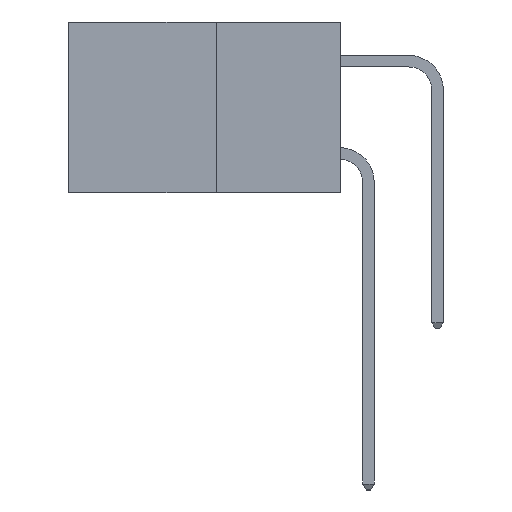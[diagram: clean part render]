
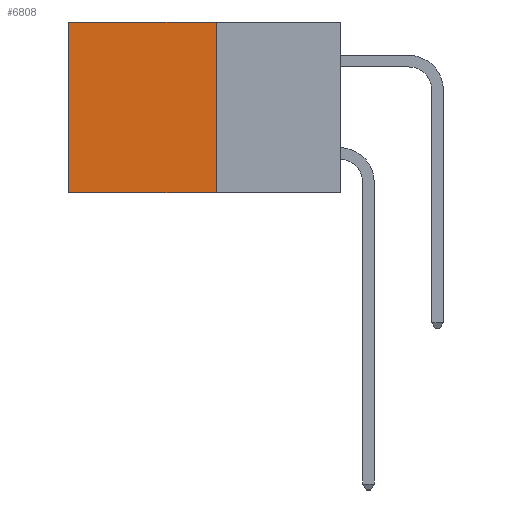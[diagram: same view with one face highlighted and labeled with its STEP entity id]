
A CAD part, left-side view. The second image highlights one B-rep face of the part: STEP entity #6808.
In plain terms, the highlighted planar face has unit normal (-1, 0, 0).
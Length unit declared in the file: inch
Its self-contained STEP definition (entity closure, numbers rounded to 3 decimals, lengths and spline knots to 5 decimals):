
#456 = EDGE_CURVE ( 'NONE', #7021, #8638, #703, .T. ) ;
#476 = VECTOR ( 'NONE', #827, 39.37008 ) ;
#616 = CARTESIAN_POINT ( 'NONE',  ( 0.277, 0.27, -0.37 ) ) ;
#703 = LINE ( 'NONE', #6790, #476 ) ;
#827 = DIRECTION ( 'NONE',  ( 0., 0., -1. ) ) ;
#1119 = VECTOR ( 'NONE', #8045, 39.37008 ) ;
#1345 = LINE ( 'NONE', #4326, #1119 ) ;
#1352 = DIRECTION ( 'NONE',  ( 0., 0., -1. ) ) ;
#1449 = LINE ( 'NONE', #4760, #7214 ) ;
#1884 = VERTEX_POINT ( 'NONE', #9195 ) ;
#2374 = DIRECTION ( 'NONE',  ( 0., 0., -1. ) ) ;
#2786 = AXIS2_PLACEMENT_3D ( 'NONE', #616, #5865, #1352 ) ;
#3178 = CARTESIAN_POINT ( 'NONE',  ( 0.277, 0.27, -0.37 ) ) ;
#3209 = DIRECTION ( 'NONE',  ( 0., 1., 0. ) ) ;
#3290 = EDGE_CURVE ( 'NONE', #1884, #8638, #1449, .T. ) ;
#4204 = ORIENTED_EDGE ( 'NONE', *, *, #7038, .F. ) ;
#4326 = CARTESIAN_POINT ( 'NONE',  ( 0.277, 0.27, 0. ) ) ;
#4546 = VECTOR ( 'NONE', #2374, 39.37008 ) ;
#4674 = FACE_OUTER_BOUND ( 'NONE', #9641, .T. ) ;
#4760 = CARTESIAN_POINT ( 'NONE',  ( 0.277, 0.27, -0.37 ) ) ;
#4793 = LINE ( 'NONE', #3178, #4546 ) ;
#4937 = VERTEX_POINT ( 'NONE', #9543 ) ;
#5019 = CARTESIAN_POINT ( 'NONE',  ( 0.277, 0.59, -0.37 ) ) ;
#5865 = DIRECTION ( 'NONE',  ( 1., 0., 0. ) ) ;
#6570 = PLANE ( 'NONE',  #2786 ) ;
#6790 = CARTESIAN_POINT ( 'NONE',  ( 0.277, 0.59, -0.37 ) ) ;
#6808 = ADVANCED_FACE ( 'NONE', ( #4674 ), #6570, .F. ) ;
#6866 = CARTESIAN_POINT ( 'NONE',  ( 0.277, 0.59, 0. ) ) ;
#7021 = VERTEX_POINT ( 'NONE', #6866 ) ;
#7038 = EDGE_CURVE ( 'NONE', #4937, #1884, #4793, .T. ) ;
#7092 = ORIENTED_EDGE ( 'NONE', *, *, #456, .T. ) ;
#7214 = VECTOR ( 'NONE', #3209, 39.37008 ) ;
#8045 = DIRECTION ( 'NONE',  ( 0., 1., 0. ) ) ;
#8115 = EDGE_CURVE ( 'NONE', #4937, #7021, #1345, .T. ) ;
#8425 = ORIENTED_EDGE ( 'NONE', *, *, #3290, .F. ) ;
#8638 = VERTEX_POINT ( 'NONE', #5019 ) ;
#9195 = CARTESIAN_POINT ( 'NONE',  ( 0.277, 0.27, -0.37 ) ) ;
#9279 = ORIENTED_EDGE ( 'NONE', *, *, #8115, .T. ) ;
#9543 = CARTESIAN_POINT ( 'NONE',  ( 0.277, 0.27, 0. ) ) ;
#9641 = EDGE_LOOP ( 'NONE', ( #7092, #8425, #4204, #9279 ) ) ;
